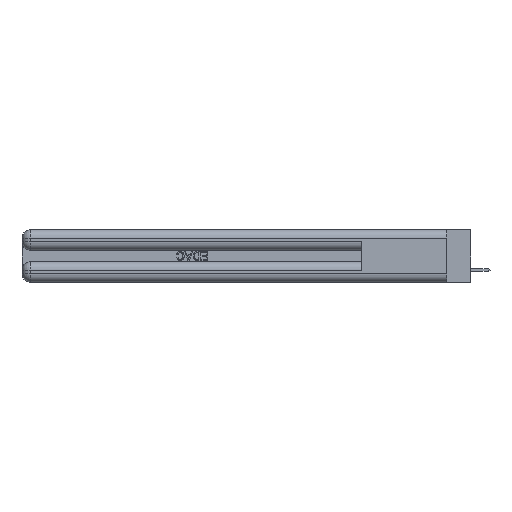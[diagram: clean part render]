
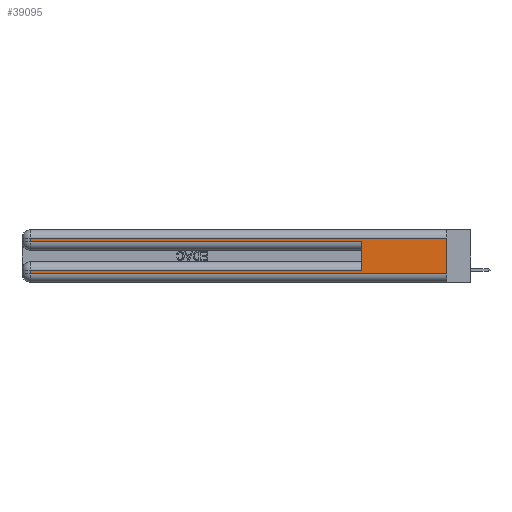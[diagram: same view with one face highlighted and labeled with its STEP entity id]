
A CAD part, left-side view. The second image highlights one B-rep face of the part: STEP entity #39095.
In plain terms, the highlighted planar face has unit normal (-1, 0, 0).
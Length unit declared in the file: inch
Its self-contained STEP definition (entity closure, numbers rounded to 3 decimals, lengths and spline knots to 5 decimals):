
#33 = VERTEX_POINT ( 'NONE', #12954 ) ;
#461 = ORIENTED_EDGE ( 'NONE', *, *, #18493, .T. ) ;
#1044 = VERTEX_POINT ( 'NONE', #22846 ) ;
#1103 = CARTESIAN_POINT ( 'NONE',  ( 0., 2.94, 0.085 ) ) ;
#1131 = DIRECTION ( 'NONE',  ( 0., 0., 1. ) ) ;
#1468 = EDGE_CURVE ( 'NONE', #33, #27704, #32623, .T. ) ;
#2280 = EDGE_CURVE ( 'NONE', #27704, #20297, #15631, .T. ) ;
#2978 = EDGE_LOOP ( 'NONE', ( #29462, #25016, #9379, #29018, #14102, #461, #4498, #8114 ) ) ;
#4498 = ORIENTED_EDGE ( 'NONE', *, *, #34366, .T. ) ;
#4909 = AXIS2_PLACEMENT_3D ( 'NONE', #38003, #31032, #11346 ) ;
#5001 = FACE_OUTER_BOUND ( 'NONE', #2978, .T. ) ;
#5440 = CARTESIAN_POINT ( 'NONE',  ( 0., 2.94, 0.31 ) ) ;
#6576 = CARTESIAN_POINT ( 'NONE',  ( 0., 2.94, 0.285 ) ) ;
#7247 = CARTESIAN_POINT ( 'NONE',  ( 0., 2.94, 0.37 ) ) ;
#8114 = ORIENTED_EDGE ( 'NONE', *, *, #19370, .T. ) ;
#9379 = ORIENTED_EDGE ( 'NONE', *, *, #2280, .T. ) ;
#10771 = CARTESIAN_POINT ( 'NONE',  ( 0., 0., 0.37 ) ) ;
#10845 = CARTESIAN_POINT ( 'NONE',  ( 0., 2.94, 0.06 ) ) ;
#11346 = DIRECTION ( 'NONE',  ( 0., 0., -1. ) ) ;
#11434 = VERTEX_POINT ( 'NONE', #10845 ) ;
#12384 = VECTOR ( 'NONE', #42265, 39.37008 ) ;
#12759 = CARTESIAN_POINT ( 'NONE',  ( 0., 2.94, 0.37 ) ) ;
#12954 = CARTESIAN_POINT ( 'NONE',  ( 0., 0., 0.31 ) ) ;
#14067 = LINE ( 'NONE', #10771, #16272 ) ;
#14102 = ORIENTED_EDGE ( 'NONE', *, *, #42044, .F. ) ;
#15572 = DIRECTION ( 'NONE',  ( 0., 1., 0. ) ) ;
#15631 = LINE ( 'NONE', #12759, #12384 ) ;
#15685 = CARTESIAN_POINT ( 'NONE',  ( 0., 0., 0.06 ) ) ;
#16272 = VECTOR ( 'NONE', #24144, 39.37008 ) ;
#16538 = VECTOR ( 'NONE', #15572, 39.37008 ) ;
#17772 = CARTESIAN_POINT ( 'NONE',  ( 0., 0.6, 0.145 ) ) ;
#18285 = VECTOR ( 'NONE', #1131, 39.37008 ) ;
#18493 = EDGE_CURVE ( 'NONE', #21919, #21791, #18560, .T. ) ;
#18560 = LINE ( 'NONE', #41705, #23942 ) ;
#19370 = EDGE_CURVE ( 'NONE', #11434, #29312, #19927, .T. ) ;
#19722 = CARTESIAN_POINT ( 'NONE',  ( 0., 0., 0.06 ) ) ;
#19927 = LINE ( 'NONE', #19722, #37891 ) ;
#20297 = VERTEX_POINT ( 'NONE', #6576 ) ;
#21630 = DIRECTION ( 'NONE',  ( 0., 1., 0. ) ) ;
#21791 = VERTEX_POINT ( 'NONE', #1103 ) ;
#21919 = VERTEX_POINT ( 'NONE', #28907 ) ;
#22143 = CARTESIAN_POINT ( 'NONE',  ( 0., 0., 0.31 ) ) ;
#22593 = DIRECTION ( 'NONE',  ( 0., -1., 0. ) ) ;
#22846 = CARTESIAN_POINT ( 'NONE',  ( 0., 0.6, 0.285 ) ) ;
#23942 = VECTOR ( 'NONE', #21630, 39.37008 ) ;
#24128 = LINE ( 'NONE', #7247, #37719 ) ;
#24144 = DIRECTION ( 'NONE',  ( 0., 0., -1. ) ) ;
#25016 = ORIENTED_EDGE ( 'NONE', *, *, #1468, .T. ) ;
#27704 = VERTEX_POINT ( 'NONE', #5440 ) ;
#28907 = CARTESIAN_POINT ( 'NONE',  ( 0., 0.6, 0.085 ) ) ;
#29018 = ORIENTED_EDGE ( 'NONE', *, *, #36052, .T. ) ;
#29312 = VERTEX_POINT ( 'NONE', #15685 ) ;
#29462 = ORIENTED_EDGE ( 'NONE', *, *, #36969, .F. ) ;
#30797 = CARTESIAN_POINT ( 'NONE',  ( 0., 0., 0.285 ) ) ;
#31032 = DIRECTION ( 'NONE',  ( 1., 0., 0. ) ) ;
#31330 = LINE ( 'NONE', #17772, #18285 ) ;
#32623 = LINE ( 'NONE', #22143, #16538 ) ;
#33520 = DIRECTION ( 'NONE',  ( 0., 0., -1. ) ) ;
#34366 = EDGE_CURVE ( 'NONE', #21791, #11434, #24128, .T. ) ;
#36052 = EDGE_CURVE ( 'NONE', #20297, #1044, #37327, .T. ) ;
#36969 = EDGE_CURVE ( 'NONE', #33, #29312, #14067, .T. ) ;
#37327 = LINE ( 'NONE', #30797, #40600 ) ;
#37719 = VECTOR ( 'NONE', #33520, 39.37008 ) ;
#37891 = VECTOR ( 'NONE', #22593, 39.37008 ) ;
#38003 = CARTESIAN_POINT ( 'NONE',  ( 0., 0., 0.37 ) ) ;
#39095 = ADVANCED_FACE ( 'NONE', ( #5001 ), #41062, .F. ) ;
#40598 = DIRECTION ( 'NONE',  ( 0., -1., 0. ) ) ;
#40600 = VECTOR ( 'NONE', #40598, 39.37008 ) ;
#41062 = PLANE ( 'NONE',  #4909 ) ;
#41705 = CARTESIAN_POINT ( 'NONE',  ( 0., 0., 0.085 ) ) ;
#42044 = EDGE_CURVE ( 'NONE', #21919, #1044, #31330, .T. ) ;
#42265 = DIRECTION ( 'NONE',  ( 0., 0., -1. ) ) ;
